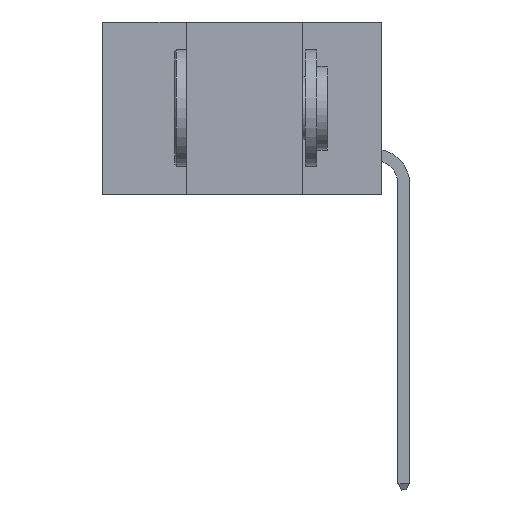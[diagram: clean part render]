
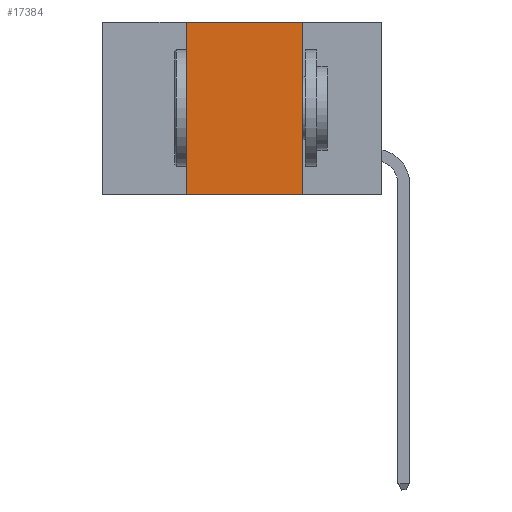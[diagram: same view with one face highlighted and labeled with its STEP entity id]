
A CAD part, left-side view. The second image highlights one B-rep face of the part: STEP entity #17384.
In plain terms, the highlighted planar face has unit normal (-1, 0, 0).
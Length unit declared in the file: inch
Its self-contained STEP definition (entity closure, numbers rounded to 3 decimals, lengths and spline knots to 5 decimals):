
#596 = PLANE ( 'NONE',  #12228 ) ;
#728 = DIRECTION ( 'NONE',  ( 0., -1., 0. ) ) ;
#3701 = CARTESIAN_POINT ( 'NONE',  ( 0., 0.6, 0. ) ) ;
#4696 = VECTOR ( 'NONE', #728, 39.37008 ) ;
#5348 = FACE_OUTER_BOUND ( 'NONE', #29892, .T. ) ;
#5450 = EDGE_CURVE ( 'NONE', #17472, #17842, #19434, .T. ) ;
#7155 = ORIENTED_EDGE ( 'NONE', *, *, #25680, .T. ) ;
#7344 = LINE ( 'NONE', #34208, #4696 ) ;
#9350 = CARTESIAN_POINT ( 'NONE',  ( 0., 0.6, 0. ) ) ;
#10555 = CARTESIAN_POINT ( 'NONE',  ( 0., 0.42, 0. ) ) ;
#12228 = AXIS2_PLACEMENT_3D ( 'NONE', #3701, #14669, #22931 ) ;
#13474 = VECTOR ( 'NONE', #17265, 39.37008 ) ;
#13501 = ORIENTED_EDGE ( 'NONE', *, *, #28927, .F. ) ;
#14362 = CARTESIAN_POINT ( 'NONE',  ( 0., 0.17, 0. ) ) ;
#14669 = DIRECTION ( 'NONE',  ( 1., 0., 0. ) ) ;
#14927 = DIRECTION ( 'NONE',  ( 0., -1., 0. ) ) ;
#15514 = VECTOR ( 'NONE', #14927, 39.37008 ) ;
#16992 = ORIENTED_EDGE ( 'NONE', *, *, #19179, .F. ) ;
#17017 = CARTESIAN_POINT ( 'NONE',  ( 0., 0.17, 0. ) ) ;
#17265 = DIRECTION ( 'NONE',  ( 0., 0., -1. ) ) ;
#17384 = ADVANCED_FACE ( 'NONE', ( #5348 ), #596, .F. ) ;
#17472 = VERTEX_POINT ( 'NONE', #20571 ) ;
#17521 = LINE ( 'NONE', #10555, #29267 ) ;
#17842 = VERTEX_POINT ( 'NONE', #17017 ) ;
#19179 = EDGE_CURVE ( 'NONE', #17842, #19712, #30894, .T. ) ;
#19434 = LINE ( 'NONE', #9350, #15514 ) ;
#19712 = VERTEX_POINT ( 'NONE', #22624 ) ;
#20571 = CARTESIAN_POINT ( 'NONE',  ( 0., 0.42, 0. ) ) ;
#21707 = DIRECTION ( 'NONE',  ( 0., 0., 1. ) ) ;
#22624 = CARTESIAN_POINT ( 'NONE',  ( 0., 0.17, -0.37 ) ) ;
#22931 = DIRECTION ( 'NONE',  ( 0., 0., -1. ) ) ;
#25496 = ORIENTED_EDGE ( 'NONE', *, *, #5450, .F. ) ;
#25680 = EDGE_CURVE ( 'NONE', #33046, #19712, #7344, .T. ) ;
#28927 = EDGE_CURVE ( 'NONE', #33046, #17472, #17521, .T. ) ;
#29267 = VECTOR ( 'NONE', #21707, 39.37008 ) ;
#29892 = EDGE_LOOP ( 'NONE', ( #16992, #25496, #13501, #7155 ) ) ;
#30894 = LINE ( 'NONE', #14362, #13474 ) ;
#33046 = VERTEX_POINT ( 'NONE', #34655 ) ;
#34208 = CARTESIAN_POINT ( 'NONE',  ( 0., 0.6, -0.37 ) ) ;
#34655 = CARTESIAN_POINT ( 'NONE',  ( 0., 0.42, -0.37 ) ) ;
